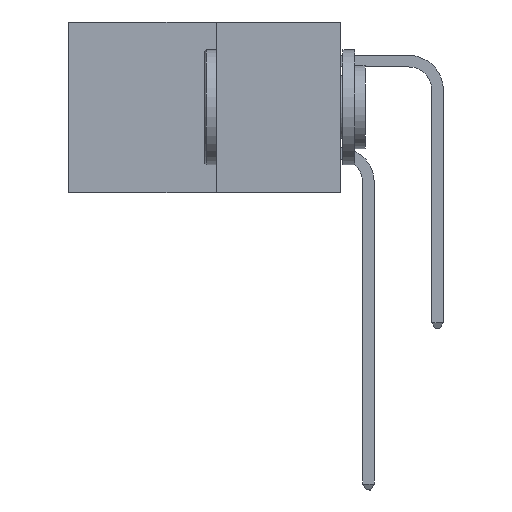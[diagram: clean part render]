
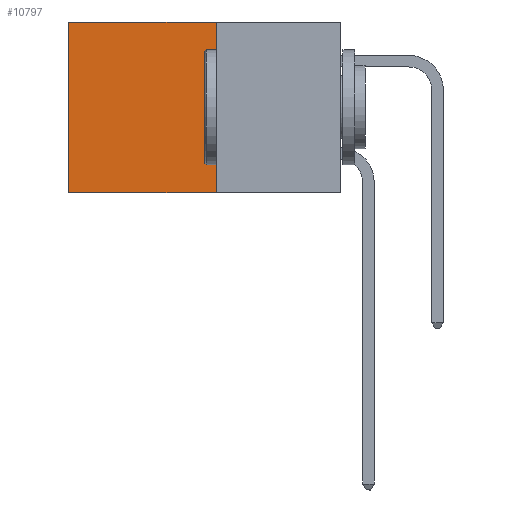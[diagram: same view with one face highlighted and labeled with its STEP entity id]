
A CAD part, left-side view. The second image highlights one B-rep face of the part: STEP entity #10797.
In plain terms, the highlighted planar face has unit normal (-1, 0, 0).
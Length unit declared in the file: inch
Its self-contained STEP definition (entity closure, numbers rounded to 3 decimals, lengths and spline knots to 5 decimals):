
#41 = CARTESIAN_POINT ( 'NONE',  ( 0.277, 0.27, -0.37 ) ) ;
#814 = VECTOR ( 'NONE', #7884, 39.37008 ) ;
#1012 = VECTOR ( 'NONE', #6005, 39.37008 ) ;
#1319 = DIRECTION ( 'NONE',  ( 1., 0., 0. ) ) ;
#1638 = VERTEX_POINT ( 'NONE', #6389 ) ;
#1790 = VERTEX_POINT ( 'NONE', #2655 ) ;
#1839 = ORIENTED_EDGE ( 'NONE', *, *, #4878, .T. ) ;
#2050 = LINE ( 'NONE', #2560, #10648 ) ;
#2151 = CARTESIAN_POINT ( 'NONE',  ( 0.277, 0.59, 0. ) ) ;
#2455 = VECTOR ( 'NONE', #8251, 39.37008 ) ;
#2560 = CARTESIAN_POINT ( 'NONE',  ( 0.277, 0.59, -0.37 ) ) ;
#2655 = CARTESIAN_POINT ( 'NONE',  ( 0.277, 0.27, 0. ) ) ;
#2922 = CARTESIAN_POINT ( 'NONE',  ( 0.277, 0.27, 0. ) ) ;
#2957 = CARTESIAN_POINT ( 'NONE',  ( 0.277, 0.27, -0.37 ) ) ;
#4358 = AXIS2_PLACEMENT_3D ( 'NONE', #10501, #1319, #7272 ) ;
#4502 = EDGE_CURVE ( 'NONE', #7480, #1638, #2050, .T. ) ;
#4673 = EDGE_CURVE ( 'NONE', #1790, #4898, #9123, .T. ) ;
#4878 = EDGE_CURVE ( 'NONE', #1790, #7480, #7820, .T. ) ;
#4898 = VERTEX_POINT ( 'NONE', #2957 ) ;
#5611 = ORIENTED_EDGE ( 'NONE', *, *, #4673, .F. ) ;
#6005 = DIRECTION ( 'NONE',  ( 0., 1., 0. ) ) ;
#6122 = FACE_OUTER_BOUND ( 'NONE', #7722, .T. ) ;
#6246 = DIRECTION ( 'NONE',  ( 0., 0., -1. ) ) ;
#6389 = CARTESIAN_POINT ( 'NONE',  ( 0.277, 0.59, -0.37 ) ) ;
#6416 = PLANE ( 'NONE',  #4358 ) ;
#7272 = DIRECTION ( 'NONE',  ( 0., 0., -1. ) ) ;
#7273 = LINE ( 'NONE', #41, #1012 ) ;
#7480 = VERTEX_POINT ( 'NONE', #2151 ) ;
#7722 = EDGE_LOOP ( 'NONE', ( #9097, #9049, #5611, #1839 ) ) ;
#7820 = LINE ( 'NONE', #2922, #814 ) ;
#7884 = DIRECTION ( 'NONE',  ( 0., 1., 0. ) ) ;
#8251 = DIRECTION ( 'NONE',  ( 0., 0., -1. ) ) ;
#8292 = EDGE_CURVE ( 'NONE', #4898, #1638, #7273, .T. ) ;
#9049 = ORIENTED_EDGE ( 'NONE', *, *, #8292, .F. ) ;
#9097 = ORIENTED_EDGE ( 'NONE', *, *, #4502, .T. ) ;
#9123 = LINE ( 'NONE', #9656, #2455 ) ;
#9656 = CARTESIAN_POINT ( 'NONE',  ( 0.277, 0.27, -0.37 ) ) ;
#10501 = CARTESIAN_POINT ( 'NONE',  ( 0.277, 0.27, -0.37 ) ) ;
#10648 = VECTOR ( 'NONE', #6246, 39.37008 ) ;
#10797 = ADVANCED_FACE ( 'NONE', ( #6122 ), #6416, .F. ) ;
